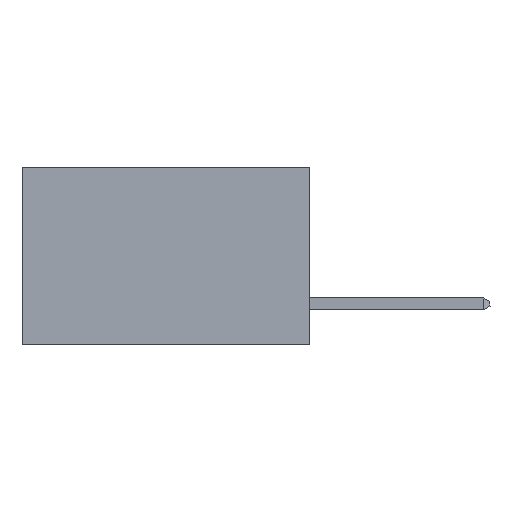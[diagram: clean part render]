
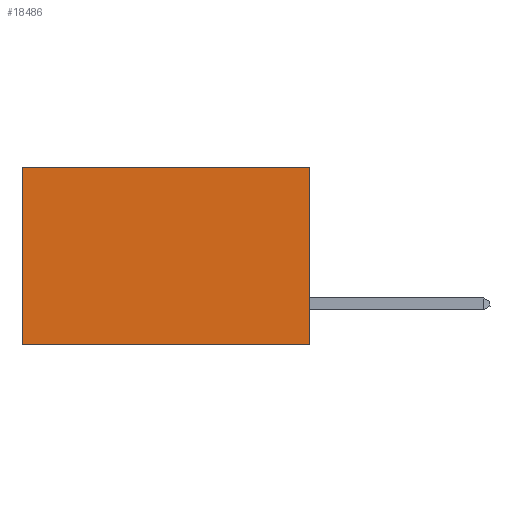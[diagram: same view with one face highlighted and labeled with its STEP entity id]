
A CAD part, left-side view. The second image highlights one B-rep face of the part: STEP entity #18486.
In plain terms, the highlighted planar face has unit normal (-1, 0, 0).
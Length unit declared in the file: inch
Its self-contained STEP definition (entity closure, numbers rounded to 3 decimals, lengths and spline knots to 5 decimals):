
#64 = VERTEX_POINT ( 'NONE', #20555 ) ;
#1153 = DIRECTION ( 'NONE',  ( 0., 0., -1. ) ) ;
#1686 = AXIS2_PLACEMENT_3D ( 'NONE', #16151, #19230, #9946 ) ;
#2124 = LINE ( 'NONE', #2314, #18680 ) ;
#2314 = CARTESIAN_POINT ( 'NONE',  ( 0.2875, 0., 0. ) ) ;
#3066 = CARTESIAN_POINT ( 'NONE',  ( 0.2875, 0., -0.37 ) ) ;
#3526 = EDGE_CURVE ( 'NONE', #64, #5716, #2124, .T. ) ;
#3561 = VECTOR ( 'NONE', #10625, 39.37008 ) ;
#3774 = VECTOR ( 'NONE', #11642, 39.37008 ) ;
#5716 = VERTEX_POINT ( 'NONE', #3066 ) ;
#6430 = VECTOR ( 'NONE', #8093, 39.37008 ) ;
#7137 = EDGE_CURVE ( 'NONE', #64, #11929, #14495, .T. ) ;
#7264 = EDGE_CURVE ( 'NONE', #5716, #13566, #20230, .T. ) ;
#7424 = CARTESIAN_POINT ( 'NONE',  ( 0.2875, 0.6, 0. ) ) ;
#8093 = DIRECTION ( 'NONE',  ( 0., 1., 0. ) ) ;
#9406 = CARTESIAN_POINT ( 'NONE',  ( 0.2875, 0.6, -0.37 ) ) ;
#9710 = FACE_OUTER_BOUND ( 'NONE', #16231, .T. ) ;
#9946 = DIRECTION ( 'NONE',  ( 0., 0., -1. ) ) ;
#10625 = DIRECTION ( 'NONE',  ( 0., 0., -1. ) ) ;
#10771 = ORIENTED_EDGE ( 'NONE', *, *, #20246, .T. ) ;
#11642 = DIRECTION ( 'NONE',  ( 0., 1., 0. ) ) ;
#11929 = VERTEX_POINT ( 'NONE', #14264 ) ;
#12381 = LINE ( 'NONE', #7424, #3561 ) ;
#13566 = VERTEX_POINT ( 'NONE', #9406 ) ;
#14264 = CARTESIAN_POINT ( 'NONE',  ( 0.2875, 0.6, 0. ) ) ;
#14495 = LINE ( 'NONE', #15933, #6430 ) ;
#14618 = PLANE ( 'NONE',  #1686 ) ;
#14689 = ORIENTED_EDGE ( 'NONE', *, *, #3526, .F. ) ;
#15045 = ORIENTED_EDGE ( 'NONE', *, *, #7264, .F. ) ;
#15063 = ORIENTED_EDGE ( 'NONE', *, *, #7137, .T. ) ;
#15933 = CARTESIAN_POINT ( 'NONE',  ( 0.2875, 0., 0. ) ) ;
#16151 = CARTESIAN_POINT ( 'NONE',  ( 0.2875, 0., 0. ) ) ;
#16231 = EDGE_LOOP ( 'NONE', ( #10771, #15045, #14689, #15063 ) ) ;
#18486 = ADVANCED_FACE ( 'NONE', ( #9710 ), #14618, .F. ) ;
#18680 = VECTOR ( 'NONE', #1153, 39.37008 ) ;
#19230 = DIRECTION ( 'NONE',  ( 1., 0., 0. ) ) ;
#20230 = LINE ( 'NONE', #20803, #3774 ) ;
#20246 = EDGE_CURVE ( 'NONE', #11929, #13566, #12381, .T. ) ;
#20555 = CARTESIAN_POINT ( 'NONE',  ( 0.2875, 0., 0. ) ) ;
#20803 = CARTESIAN_POINT ( 'NONE',  ( 0.2875, 0., -0.37 ) ) ;
